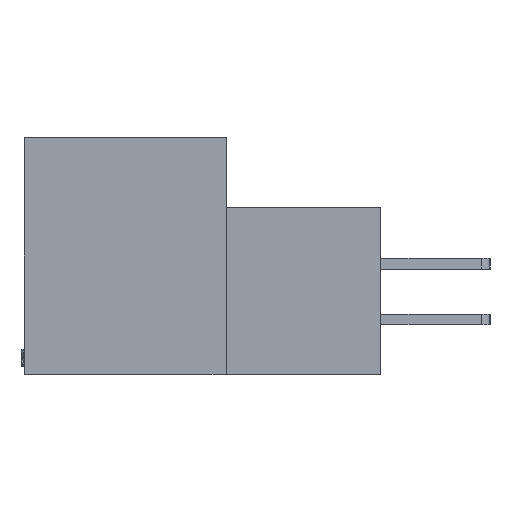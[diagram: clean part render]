
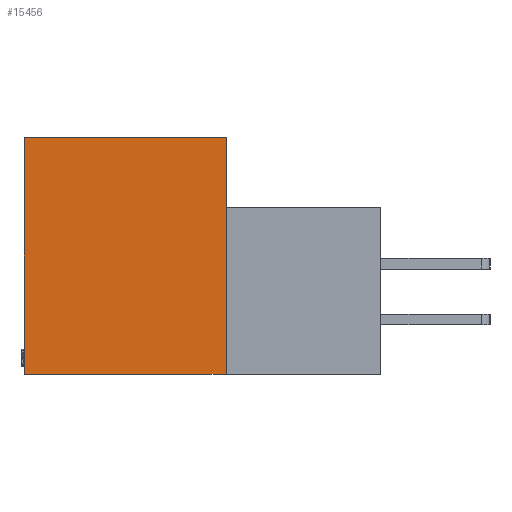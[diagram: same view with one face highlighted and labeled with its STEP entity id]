
A CAD part, left-side view. The second image highlights one B-rep face of the part: STEP entity #15456.
In plain terms, the highlighted planar face has unit normal (-1, 0, 0).
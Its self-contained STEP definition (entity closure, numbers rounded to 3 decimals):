
#240 = VECTOR ( 'NONE', #13222, 1000. ) ;
#317 = CARTESIAN_POINT ( 'NONE',  ( 0., 11.506, -13.487 ) ) ;
#1025 = CARTESIAN_POINT ( 'NONE',  ( 0., 11.506, -13.487 ) ) ;
#1485 = VECTOR ( 'NONE', #4623, 1000. ) ;
#3124 = CARTESIAN_POINT ( 'NONE',  ( 0., 0., -13.487 ) ) ;
#3461 = LINE ( 'NONE', #11123, #240 ) ;
#4215 = DIRECTION ( 'NONE',  ( 0., 0., 1. ) ) ;
#4623 = DIRECTION ( 'NONE',  ( 0., -1., 0. ) ) ;
#4888 = CARTESIAN_POINT ( 'NONE',  ( 0., 0., 0. ) ) ;
#5450 = VERTEX_POINT ( 'NONE', #18150 ) ;
#5832 = DIRECTION ( 'NONE',  ( 0., 0., -1. ) ) ;
#6355 = VECTOR ( 'NONE', #4215, 1000. ) ;
#6460 = ORIENTED_EDGE ( 'NONE', *, *, #20220, .F. ) ;
#8717 = VERTEX_POINT ( 'NONE', #3124 ) ;
#10933 = ORIENTED_EDGE ( 'NONE', *, *, #25387, .F. ) ;
#11123 = CARTESIAN_POINT ( 'NONE',  ( 0., 0., 0. ) ) ;
#12655 = CARTESIAN_POINT ( 'NONE',  ( 0., 0., 0. ) ) ;
#13222 = DIRECTION ( 'NONE',  ( 0., 0., -1. ) ) ;
#13845 = EDGE_CURVE ( 'NONE', #16342, #8717, #3461, .T. ) ;
#14235 = LINE ( 'NONE', #25000, #1485 ) ;
#14807 = VERTEX_POINT ( 'NONE', #1025 ) ;
#15456 = ADVANCED_FACE ( 'NONE', ( #21843 ), #26219, .F. ) ;
#16342 = VERTEX_POINT ( 'NONE', #4888 ) ;
#17350 = DIRECTION ( 'NONE',  ( 1., 0., 0. ) ) ;
#18150 = CARTESIAN_POINT ( 'NONE',  ( 0., 11.506, 0. ) ) ;
#18800 = CARTESIAN_POINT ( 'NONE',  ( 0., -8.814, -13.487 ) ) ;
#18993 = DIRECTION ( 'NONE',  ( 0., 1., 0. ) ) ;
#20220 = EDGE_CURVE ( 'NONE', #5450, #16342, #14235, .T. ) ;
#21564 = EDGE_CURVE ( 'NONE', #14807, #5450, #23426, .T. ) ;
#21843 = FACE_OUTER_BOUND ( 'NONE', #25214, .T. ) ;
#23274 = LINE ( 'NONE', #18800, #28222 ) ;
#23426 = LINE ( 'NONE', #317, #6355 ) ;
#24758 = ORIENTED_EDGE ( 'NONE', *, *, #13845, .F. ) ;
#25000 = CARTESIAN_POINT ( 'NONE',  ( 0., 11.506, 0. ) ) ;
#25214 = EDGE_LOOP ( 'NONE', ( #10933, #24758, #6460, #25759 ) ) ;
#25387 = EDGE_CURVE ( 'NONE', #8717, #14807, #23274, .T. ) ;
#25759 = ORIENTED_EDGE ( 'NONE', *, *, #21564, .F. ) ;
#26219 = PLANE ( 'NONE',  #26222 ) ;
#26222 = AXIS2_PLACEMENT_3D ( 'NONE', #12655, #17350, #5832 ) ;
#28222 = VECTOR ( 'NONE', #18993, 1000. ) ;
